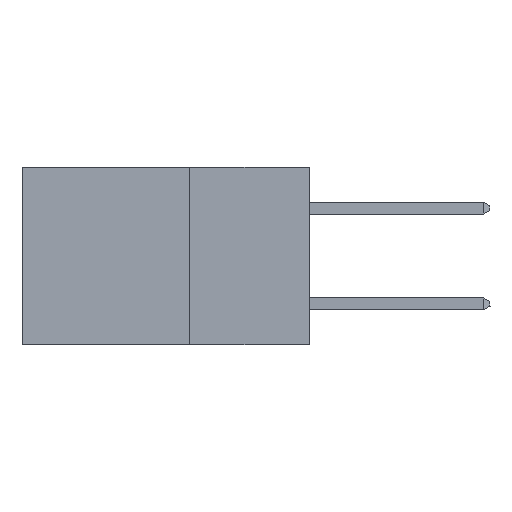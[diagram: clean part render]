
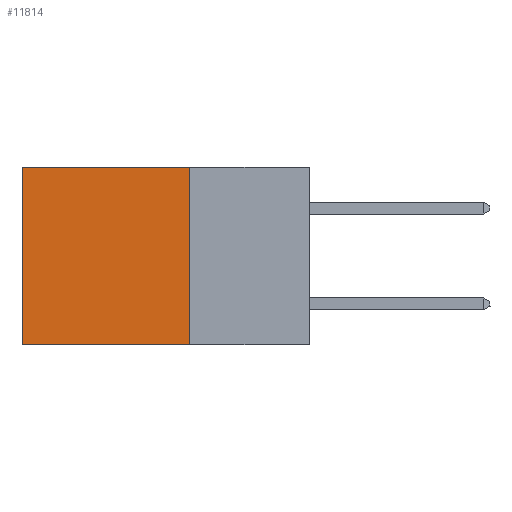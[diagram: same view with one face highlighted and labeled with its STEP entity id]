
A CAD part, left-side view. The second image highlights one B-rep face of the part: STEP entity #11814.
In plain terms, the highlighted planar face has unit normal (-1, 0, 0).
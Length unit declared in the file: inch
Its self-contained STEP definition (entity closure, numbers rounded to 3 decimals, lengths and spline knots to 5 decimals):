
#2432 = EDGE_CURVE ( 'NONE', #14117, #9182, #8044, .T. ) ;
#2453 = ORIENTED_EDGE ( 'NONE', *, *, #2432, .T. ) ;
#2685 = LINE ( 'NONE', #23701, #15044 ) ;
#2954 = DIRECTION ( 'NONE',  ( 0., 1., 0. ) ) ;
#4342 = VECTOR ( 'NONE', #2954, 39.37008 ) ;
#6712 = EDGE_CURVE ( 'NONE', #14117, #29409, #2685, .T. ) ;
#8044 = LINE ( 'NONE', #16057, #32162 ) ;
#8923 = PLANE ( 'NONE',  #27589 ) ;
#9182 = VERTEX_POINT ( 'NONE', #36598 ) ;
#9190 = DIRECTION ( 'NONE',  ( 1., 0., 0. ) ) ;
#9703 = CARTESIAN_POINT ( 'NONE',  ( 0.2875, 0.25, -0.37 ) ) ;
#11814 = ADVANCED_FACE ( 'NONE', ( #13650 ), #8923, .F. ) ;
#13650 = FACE_OUTER_BOUND ( 'NONE', #15998, .T. ) ;
#14117 = VERTEX_POINT ( 'NONE', #32486 ) ;
#14771 = DIRECTION ( 'NONE',  ( 0., 0., -1. ) ) ;
#15044 = VECTOR ( 'NONE', #14771, 39.37008 ) ;
#15998 = EDGE_LOOP ( 'NONE', ( #20948, #24427, #40683, #2453 ) ) ;
#16057 = CARTESIAN_POINT ( 'NONE',  ( 0.2875, 0.25, 0. ) ) ;
#19823 = DIRECTION ( 'NONE',  ( 0., 0., -1. ) ) ;
#20948 = ORIENTED_EDGE ( 'NONE', *, *, #24978, .T. ) ;
#21223 = EDGE_CURVE ( 'NONE', #29409, #23082, #28926, .T. ) ;
#21288 = CARTESIAN_POINT ( 'NONE',  ( 0.2875, 0.25, 0. ) ) ;
#22711 = CARTESIAN_POINT ( 'NONE',  ( 0.2875, 0.6, 0. ) ) ;
#23082 = VERTEX_POINT ( 'NONE', #28410 ) ;
#23653 = VECTOR ( 'NONE', #19823, 39.37008 ) ;
#23701 = CARTESIAN_POINT ( 'NONE',  ( 0.2875, 0.25, 0. ) ) ;
#24427 = ORIENTED_EDGE ( 'NONE', *, *, #21223, .F. ) ;
#24598 = CARTESIAN_POINT ( 'NONE',  ( 0.2875, 0.25, -0.37 ) ) ;
#24978 = EDGE_CURVE ( 'NONE', #9182, #23082, #32013, .T. ) ;
#26208 = DIRECTION ( 'NONE',  ( 0., 1., 0. ) ) ;
#27589 = AXIS2_PLACEMENT_3D ( 'NONE', #21288, #9190, #37395 ) ;
#28410 = CARTESIAN_POINT ( 'NONE',  ( 0.2875, 0.6, -0.37 ) ) ;
#28926 = LINE ( 'NONE', #9703, #4342 ) ;
#29409 = VERTEX_POINT ( 'NONE', #24598 ) ;
#32013 = LINE ( 'NONE', #22711, #23653 ) ;
#32162 = VECTOR ( 'NONE', #26208, 39.37008 ) ;
#32486 = CARTESIAN_POINT ( 'NONE',  ( 0.2875, 0.25, 0. ) ) ;
#36598 = CARTESIAN_POINT ( 'NONE',  ( 0.2875, 0.6, 0. ) ) ;
#37395 = DIRECTION ( 'NONE',  ( 0., 0., -1. ) ) ;
#40683 = ORIENTED_EDGE ( 'NONE', *, *, #6712, .F. ) ;
